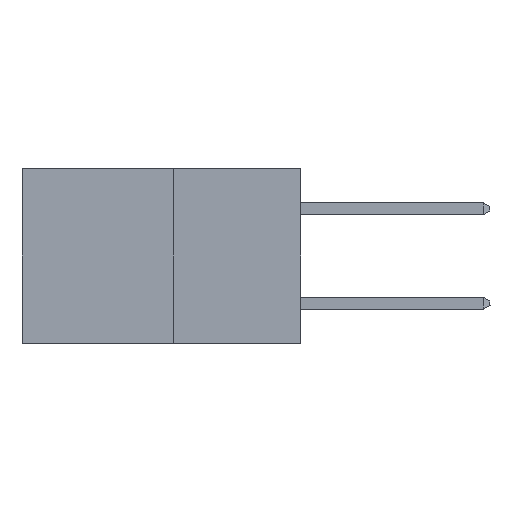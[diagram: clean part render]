
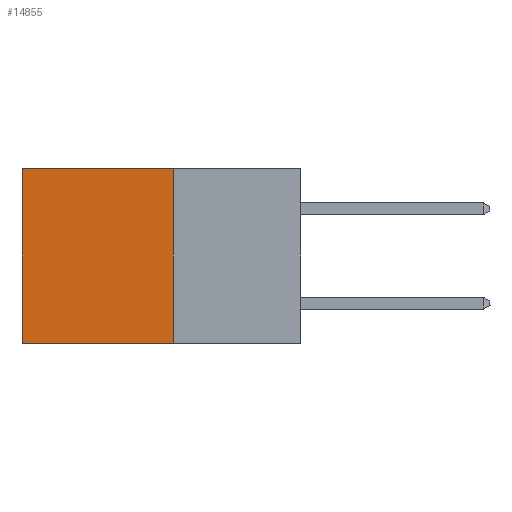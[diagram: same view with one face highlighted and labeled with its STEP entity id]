
A CAD part, left-side view. The second image highlights one B-rep face of the part: STEP entity #14855.
In plain terms, the highlighted planar face has unit normal (-1, 0, 0).
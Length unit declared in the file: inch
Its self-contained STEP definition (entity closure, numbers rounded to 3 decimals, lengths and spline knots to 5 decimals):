
#317 = ORIENTED_EDGE ( 'NONE', *, *, #7782, .F. ) ;
#438 = CARTESIAN_POINT ( 'NONE',  ( 0.277, 0.59, -0.37 ) ) ;
#549 = VECTOR ( 'NONE', #1728, 39.37008 ) ;
#1728 = DIRECTION ( 'NONE',  ( 0., 1., 0. ) ) ;
#1816 = VERTEX_POINT ( 'NONE', #6593 ) ;
#1936 = CARTESIAN_POINT ( 'NONE',  ( 0.277, 0.27, -0.37 ) ) ;
#2108 = CARTESIAN_POINT ( 'NONE',  ( 0.277, 0.59, -0.37 ) ) ;
#2515 = CARTESIAN_POINT ( 'NONE',  ( 0.277, 0.27, 0. ) ) ;
#2616 = DIRECTION ( 'NONE',  ( 0., 0., -1. ) ) ;
#2921 = LINE ( 'NONE', #438, #8739 ) ;
#3346 = VECTOR ( 'NONE', #2616, 39.37008 ) ;
#3685 = ORIENTED_EDGE ( 'NONE', *, *, #9235, .T. ) ;
#3805 = CARTESIAN_POINT ( 'NONE',  ( 0.277, 0.27, -0.37 ) ) ;
#3927 = EDGE_CURVE ( 'NONE', #13339, #6163, #9513, .T. ) ;
#4269 = CARTESIAN_POINT ( 'NONE',  ( 0.277, 0.27, -0.37 ) ) ;
#4891 = FACE_OUTER_BOUND ( 'NONE', #14238, .T. ) ;
#6163 = VERTEX_POINT ( 'NONE', #2108 ) ;
#6593 = CARTESIAN_POINT ( 'NONE',  ( 0.277, 0.59, 0. ) ) ;
#6772 = DIRECTION ( 'NONE',  ( 0., 0., -1. ) ) ;
#7606 = VECTOR ( 'NONE', #15047, 39.37008 ) ;
#7782 = EDGE_CURVE ( 'NONE', #13008, #13339, #12680, .T. ) ;
#7921 = CARTESIAN_POINT ( 'NONE',  ( 0.277, 0.27, 0. ) ) ;
#8255 = ORIENTED_EDGE ( 'NONE', *, *, #3927, .F. ) ;
#8739 = VECTOR ( 'NONE', #12162, 39.37008 ) ;
#9235 = EDGE_CURVE ( 'NONE', #1816, #6163, #2921, .T. ) ;
#9479 = ORIENTED_EDGE ( 'NONE', *, *, #14862, .T. ) ;
#9513 = LINE ( 'NONE', #1936, #549 ) ;
#10737 = LINE ( 'NONE', #7921, #7606 ) ;
#11433 = PLANE ( 'NONE',  #12240 ) ;
#12162 = DIRECTION ( 'NONE',  ( 0., 0., -1. ) ) ;
#12240 = AXIS2_PLACEMENT_3D ( 'NONE', #12592, #13856, #6772 ) ;
#12592 = CARTESIAN_POINT ( 'NONE',  ( 0.277, 0.27, -0.37 ) ) ;
#12680 = LINE ( 'NONE', #3805, #3346 ) ;
#13008 = VERTEX_POINT ( 'NONE', #2515 ) ;
#13339 = VERTEX_POINT ( 'NONE', #4269 ) ;
#13856 = DIRECTION ( 'NONE',  ( 1., 0., 0. ) ) ;
#14238 = EDGE_LOOP ( 'NONE', ( #3685, #8255, #317, #9479 ) ) ;
#14855 = ADVANCED_FACE ( 'NONE', ( #4891 ), #11433, .F. ) ;
#14862 = EDGE_CURVE ( 'NONE', #13008, #1816, #10737, .T. ) ;
#15047 = DIRECTION ( 'NONE',  ( 0., 1., 0. ) ) ;
